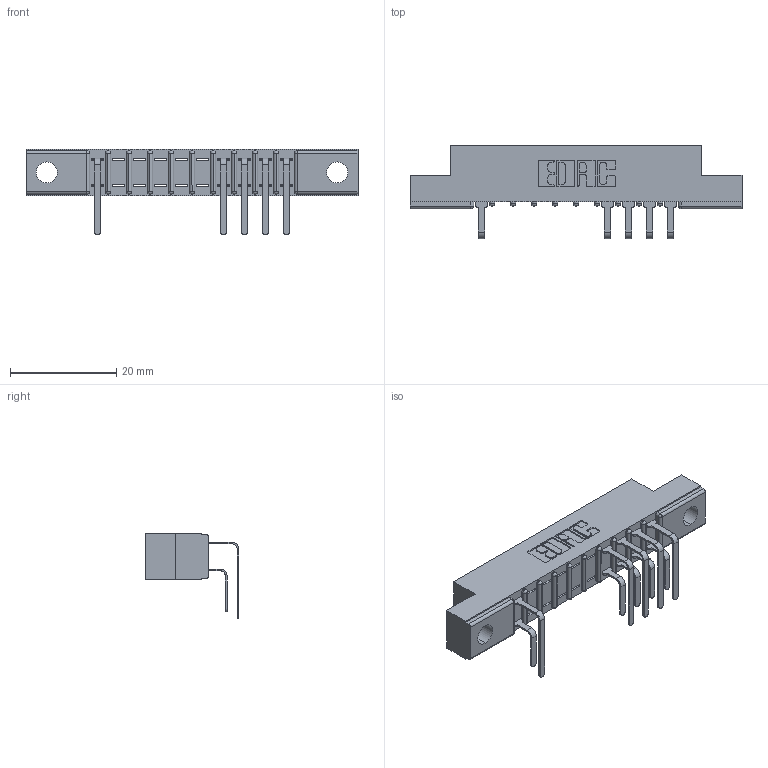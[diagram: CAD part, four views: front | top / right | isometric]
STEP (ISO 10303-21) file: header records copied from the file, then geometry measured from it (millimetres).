
FILE_DESCRIPTION (( 'STEP AP203' ), '1' );
FILE_NAME ('307-010-559-104.STEP', '2018-08-02T21:13:59', ( '' ), ( '' ), 'SwSTEP 2.0', 'SolidWorks 2016', '' );
FILE_SCHEMA (( 'CONFIG_CONTROL_DESIGN' ));
Length unit declared in the file: inch
Products named in the file (4): 307-010-559-104; 307 Part_.156 Dia Mounting Holes; 307-290-001_558 559 - 1 (Single); 307-290-001_559 - 2 (Single)
Assembly tree (11 placements, depth 2):
  307-010-559-104
    307 Part_.156 Dia Mounting Holes
    307-290-001_558 559 - 1 (Single)  x5
    307-290-001_559 - 2 (Single)  x5
Bounding box: 62.64 x 17.69 x 16.08 mm (x, y, z)
Volume: 3907.3 mm3; surface area: 5649 mm2
Topology: 11 solids, 11 shells, 743 faces, 2099 edges, 1354 vertices
Faces by surface type: plane 474, cylinder 247, sphere 22
Entity records: 14383 total; most frequent: CARTESIAN_POINT 2412, ORIENTED_EDGE 2394, DIRECTION 2357, EDGE_CURVE 1197, LINE 911, VECTOR 911, VERTEX_POINT 778, AXIS2_PLACEMENT_3D 723
